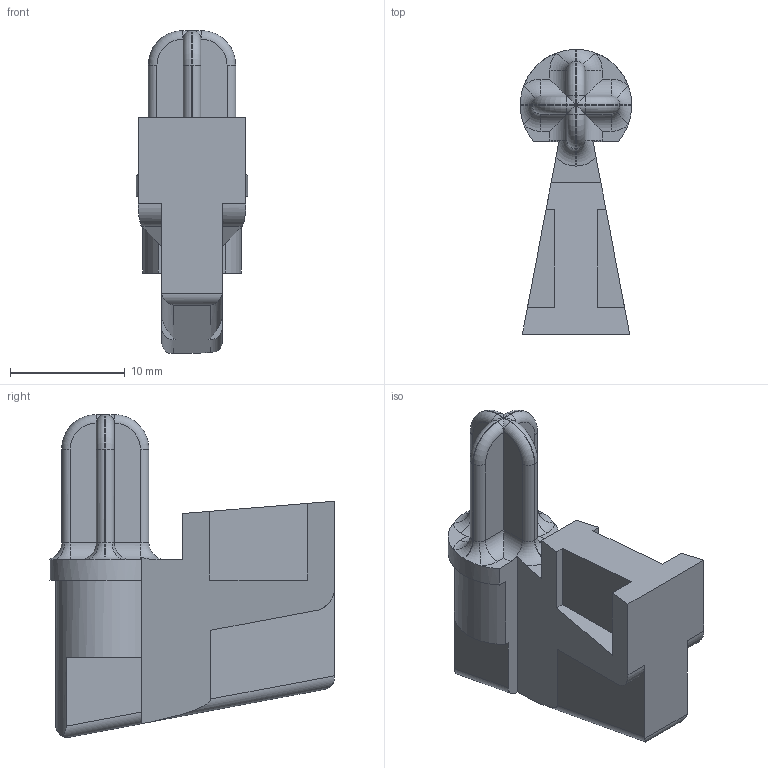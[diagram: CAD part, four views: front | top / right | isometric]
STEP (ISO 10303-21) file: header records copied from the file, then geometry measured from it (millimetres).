
FILE_DESCRIPTION(/* description */ (''),/* implementation_level */ '2;1');
FILE_NAME(/* name */ 'Follower v6.step',/* time_stamp */ '2020-03-23T02:04:45-04:00',/* author */ (''),/* organization */ (''),/* preprocessor_version */ 'ST-DEVELOPER v18',/* originating_system */ 'Autodesk Translation Framework v8.12.0.6',/* authorisation */ '');
FILE_SCHEMA (('AUTOMOTIVE_DESIGN { 1 0 10303 214 3 1 1 }'));
Length unit declared in the file: millimetre
Products named in the file (1): Follower
Bounding box: 9.7 x 24.8 x 28.09 mm (x, y, z)
Volume: 2338.1 mm3; surface area: 1697.5 mm2
Topology: 1 solids, 1 shells, 110 faces, 278 edges, 170 vertices
Faces by surface type: plane 44, cylinder 43, torus 22, bspline 1
Entity records: 3414 total; most frequent: CARTESIAN_POINT 691, DIRECTION 593, ORIENTED_EDGE 556, EDGE_CURVE 278, AXIS2_PLACEMENT_3D 222, VERTEX_POINT 170, LINE 149, VECTOR 149
